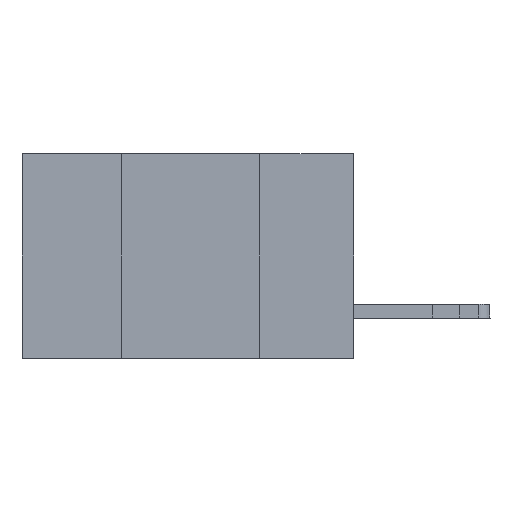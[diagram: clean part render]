
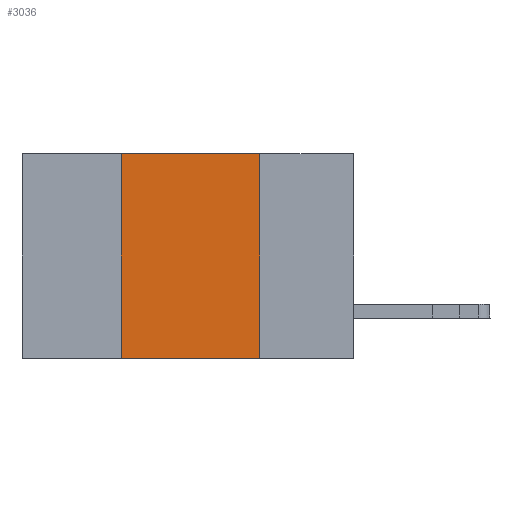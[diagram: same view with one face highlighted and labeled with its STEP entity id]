
A CAD part, left-side view. The second image highlights one B-rep face of the part: STEP entity #3036.
In plain terms, the highlighted planar face has unit normal (-1, 0, 0).
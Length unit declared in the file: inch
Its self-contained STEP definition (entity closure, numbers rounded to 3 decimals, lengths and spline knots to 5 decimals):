
#41 = EDGE_LOOP ( 'NONE', ( #6826, #13613, #4156, #12098 ) ) ;
#2513 = VECTOR ( 'NONE', #25113, 39.37008 ) ;
#2730 = VECTOR ( 'NONE', #16825, 39.37008 ) ;
#2890 = DIRECTION ( 'NONE',  ( 0., -1., 0. ) ) ;
#3036 = ADVANCED_FACE ( 'NONE', ( #11328 ), #9700, .F. ) ;
#3273 = LINE ( 'NONE', #17479, #13749 ) ;
#4156 = ORIENTED_EDGE ( 'NONE', *, *, #19024, .F. ) ;
#5902 = CARTESIAN_POINT ( 'NONE',  ( 0., 0.17, 0. ) ) ;
#6396 = CARTESIAN_POINT ( 'NONE',  ( 0., 0.6, -0.37 ) ) ;
#6495 = EDGE_CURVE ( 'NONE', #21544, #20679, #3273, .T. ) ;
#6826 = ORIENTED_EDGE ( 'NONE', *, *, #17070, .F. ) ;
#8582 = DIRECTION ( 'NONE',  ( 0., 0., -1. ) ) ;
#8757 = VERTEX_POINT ( 'NONE', #24282 ) ;
#9700 = PLANE ( 'NONE',  #17445 ) ;
#10052 = CARTESIAN_POINT ( 'NONE',  ( 0., 0.42, -0.37 ) ) ;
#10231 = CARTESIAN_POINT ( 'NONE',  ( 0., 0.17, 0. ) ) ;
#10370 = CARTESIAN_POINT ( 'NONE',  ( 0., 0.42, 0. ) ) ;
#10481 = VERTEX_POINT ( 'NONE', #10052 ) ;
#10639 = CARTESIAN_POINT ( 'NONE',  ( 0., 0.42, 0. ) ) ;
#11328 = FACE_OUTER_BOUND ( 'NONE', #41, .T. ) ;
#12098 = ORIENTED_EDGE ( 'NONE', *, *, #12750, .T. ) ;
#12750 = EDGE_CURVE ( 'NONE', #10481, #8757, #24448, .T. ) ;
#13613 = ORIENTED_EDGE ( 'NONE', *, *, #6495, .F. ) ;
#13749 = VECTOR ( 'NONE', #2890, 39.37008 ) ;
#13901 = DIRECTION ( 'NONE',  ( 0., 0., -1. ) ) ;
#16825 = DIRECTION ( 'NONE',  ( 0., -1., 0. ) ) ;
#17070 = EDGE_CURVE ( 'NONE', #20679, #8757, #17755, .T. ) ;
#17445 = AXIS2_PLACEMENT_3D ( 'NONE', #18167, #24452, #13901 ) ;
#17479 = CARTESIAN_POINT ( 'NONE',  ( 0., 0.6, 0. ) ) ;
#17755 = LINE ( 'NONE', #10231, #22683 ) ;
#18167 = CARTESIAN_POINT ( 'NONE',  ( 0., 0.6, 0. ) ) ;
#19024 = EDGE_CURVE ( 'NONE', #10481, #21544, #24891, .T. ) ;
#20679 = VERTEX_POINT ( 'NONE', #5902 ) ;
#21544 = VERTEX_POINT ( 'NONE', #10639 ) ;
#22683 = VECTOR ( 'NONE', #8582, 39.37008 ) ;
#24282 = CARTESIAN_POINT ( 'NONE',  ( 0., 0.17, -0.37 ) ) ;
#24448 = LINE ( 'NONE', #6396, #2730 ) ;
#24452 = DIRECTION ( 'NONE',  ( 1., 0., 0. ) ) ;
#24891 = LINE ( 'NONE', #10370, #2513 ) ;
#25113 = DIRECTION ( 'NONE',  ( 0., 0., 1. ) ) ;
